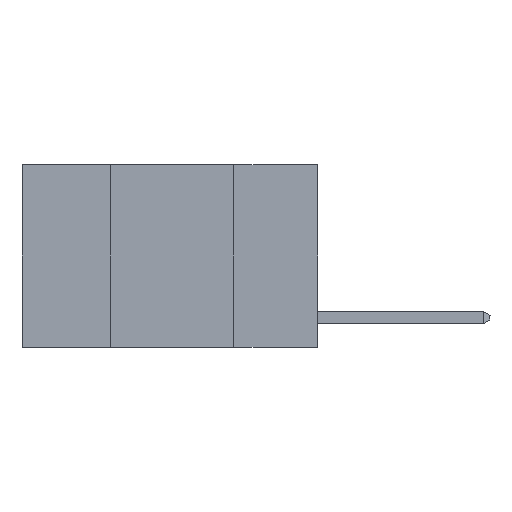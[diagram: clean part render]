
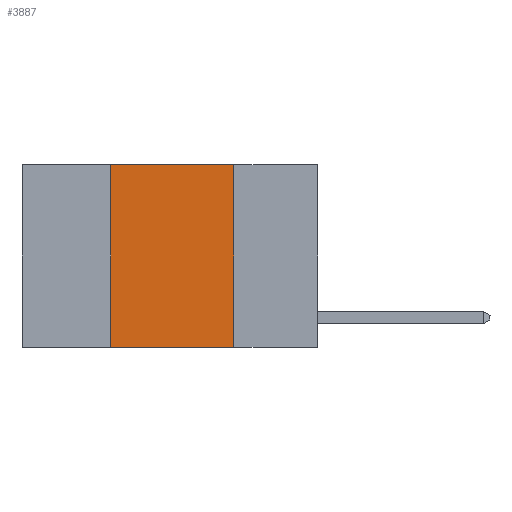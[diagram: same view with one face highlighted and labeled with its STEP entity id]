
A CAD part, left-side view. The second image highlights one B-rep face of the part: STEP entity #3887.
In plain terms, the highlighted planar face has unit normal (-1, 0, 0).
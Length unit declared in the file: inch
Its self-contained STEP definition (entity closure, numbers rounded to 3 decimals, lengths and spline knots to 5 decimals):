
#8 = CARTESIAN_POINT ( 'NONE',  ( 0., 0.42, 0. ) ) ;
#273 = VERTEX_POINT ( 'NONE', #2300 ) ;
#685 = ORIENTED_EDGE ( 'NONE', *, *, #12574, .T. ) ;
#951 = EDGE_CURVE ( 'NONE', #4429, #5661, #2356, .T. ) ;
#1098 = CARTESIAN_POINT ( 'NONE',  ( 0., 0.42, 0. ) ) ;
#1170 = LINE ( 'NONE', #1098, #12395 ) ;
#1202 = DIRECTION ( 'NONE',  ( 0., -1., 0. ) ) ;
#1436 = DIRECTION ( 'NONE',  ( 0., 0., -1. ) ) ;
#1630 = VECTOR ( 'NONE', #1436, 39.37008 ) ;
#1708 = LINE ( 'NONE', #10046, #10352 ) ;
#2191 = LINE ( 'NONE', #7469, #13812 ) ;
#2300 = CARTESIAN_POINT ( 'NONE',  ( 0., 0.42, -0.37 ) ) ;
#2356 = LINE ( 'NONE', #6800, #1630 ) ;
#2757 = CARTESIAN_POINT ( 'NONE',  ( 0., 0.17, -0.37 ) ) ;
#3624 = DIRECTION ( 'NONE',  ( 0., 0., -1. ) ) ;
#3887 = ADVANCED_FACE ( 'NONE', ( #9107 ), #5872, .F. ) ;
#3943 = ORIENTED_EDGE ( 'NONE', *, *, #10021, .F. ) ;
#4279 = EDGE_CURVE ( 'NONE', #6847, #4429, #2191, .T. ) ;
#4429 = VERTEX_POINT ( 'NONE', #12071 ) ;
#5395 = DIRECTION ( 'NONE',  ( 0., 0., 1. ) ) ;
#5506 = ORIENTED_EDGE ( 'NONE', *, *, #4279, .F. ) ;
#5661 = VERTEX_POINT ( 'NONE', #2757 ) ;
#5872 = PLANE ( 'NONE',  #13817 ) ;
#6800 = CARTESIAN_POINT ( 'NONE',  ( 0., 0.17, 0. ) ) ;
#6847 = VERTEX_POINT ( 'NONE', #8 ) ;
#7070 = DIRECTION ( 'NONE',  ( 0., -1., 0. ) ) ;
#7469 = CARTESIAN_POINT ( 'NONE',  ( 0., 0.6, 0. ) ) ;
#7971 = DIRECTION ( 'NONE',  ( 1., 0., 0. ) ) ;
#9107 = FACE_OUTER_BOUND ( 'NONE', #10714, .T. ) ;
#10021 = EDGE_CURVE ( 'NONE', #273, #6847, #1170, .T. ) ;
#10046 = CARTESIAN_POINT ( 'NONE',  ( 0., 0.6, -0.37 ) ) ;
#10152 = ORIENTED_EDGE ( 'NONE', *, *, #951, .F. ) ;
#10352 = VECTOR ( 'NONE', #7070, 39.37008 ) ;
#10714 = EDGE_LOOP ( 'NONE', ( #10152, #5506, #3943, #685 ) ) ;
#12071 = CARTESIAN_POINT ( 'NONE',  ( 0., 0.17, 0. ) ) ;
#12395 = VECTOR ( 'NONE', #5395, 39.37008 ) ;
#12574 = EDGE_CURVE ( 'NONE', #273, #5661, #1708, .T. ) ;
#13315 = CARTESIAN_POINT ( 'NONE',  ( 0., 0.6, 0. ) ) ;
#13812 = VECTOR ( 'NONE', #1202, 39.37008 ) ;
#13817 = AXIS2_PLACEMENT_3D ( 'NONE', #13315, #7971, #3624 ) ;
